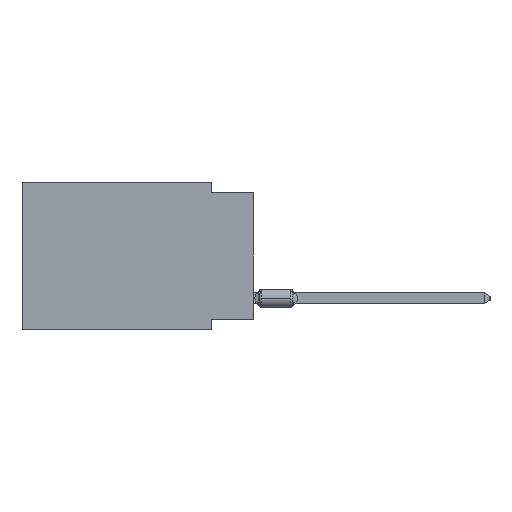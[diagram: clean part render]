
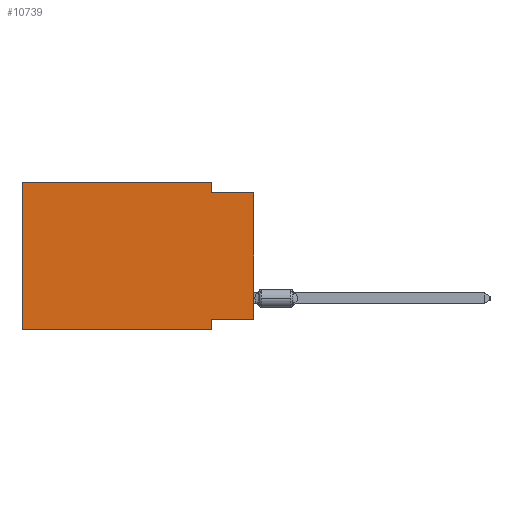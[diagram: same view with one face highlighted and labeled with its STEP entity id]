
A CAD part, left-side view. The second image highlights one B-rep face of the part: STEP entity #10739.
In plain terms, the highlighted planar face has unit normal (-1, 0, 0).
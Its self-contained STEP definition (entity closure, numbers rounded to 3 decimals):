
#89 = EDGE_CURVE ( 'NONE', #37740, #52494, #34075, .T. ) ;
#1620 = VERTEX_POINT ( 'NONE', #48824 ) ;
#2549 = DIRECTION ( 'NONE',  ( 0., 0., -1. ) ) ;
#2616 = DIRECTION ( 'NONE',  ( 0., 1., 0. ) ) ;
#3438 = VECTOR ( 'NONE', #48054, 1000. ) ;
#3888 = LINE ( 'NONE', #55420, #17510 ) ;
#4563 = ORIENTED_EDGE ( 'NONE', *, *, #40846, .T. ) ;
#4579 = DIRECTION ( 'NONE',  ( 0., 0., 1. ) ) ;
#4786 = EDGE_CURVE ( 'NONE', #1620, #22868, #50699, .T. ) ;
#5917 = ORIENTED_EDGE ( 'NONE', *, *, #14715, .F. ) ;
#9304 = EDGE_LOOP ( 'NONE', ( #4563, #17468, #33522, #39789, #30002, #59952, #5917, #35940 ) ) ;
#9480 = VECTOR ( 'NONE', #9847, 1000. ) ;
#9700 = LINE ( 'NONE', #28296, #36802 ) ;
#9847 = DIRECTION ( 'NONE',  ( 0., 0., -1. ) ) ;
#10182 = CARTESIAN_POINT ( 'NONE',  ( 0., 13.97, -8.89 ) ) ;
#10471 = CARTESIAN_POINT ( 'NONE',  ( 0., 2.54, 0. ) ) ;
#10739 = ADVANCED_FACE ( 'NONE', ( #45367 ), #35446, .F. ) ;
#10779 = CARTESIAN_POINT ( 'NONE',  ( 0., 13.97, 0. ) ) ;
#11839 = DIRECTION ( 'NONE',  ( 1., 0., 0. ) ) ;
#14715 = EDGE_CURVE ( 'NONE', #22868, #53963, #22720, .T. ) ;
#15828 = EDGE_CURVE ( 'NONE', #37740, #53963, #25347, .T. ) ;
#17404 = CARTESIAN_POINT ( 'NONE',  ( 0., 13.97, 0. ) ) ;
#17440 = AXIS2_PLACEMENT_3D ( 'NONE', #17404, #11839, #2549 ) ;
#17464 = DIRECTION ( 'NONE',  ( 0., 0., -1. ) ) ;
#17468 = ORIENTED_EDGE ( 'NONE', *, *, #26777, .F. ) ;
#17510 = VECTOR ( 'NONE', #56039, 1000. ) ;
#22555 = CARTESIAN_POINT ( 'NONE',  ( 0., 2.54, 0. ) ) ;
#22720 = LINE ( 'NONE', #26766, #59843 ) ;
#22868 = VERTEX_POINT ( 'NONE', #36745 ) ;
#25347 = LINE ( 'NONE', #10182, #3438 ) ;
#26766 = CARTESIAN_POINT ( 'NONE',  ( 0., 2.54, -8.89 ) ) ;
#26777 = EDGE_CURVE ( 'NONE', #56768, #56970, #3888, .T. ) ;
#27705 = VECTOR ( 'NONE', #4579, 1000. ) ;
#28296 = CARTESIAN_POINT ( 'NONE',  ( 0., 0., 0. ) ) ;
#28320 = CARTESIAN_POINT ( 'NONE',  ( 0., 2.54, -8.89 ) ) ;
#30002 = ORIENTED_EDGE ( 'NONE', *, *, #89, .F. ) ;
#30354 = CARTESIAN_POINT ( 'NONE',  ( 0., 0., -0.635 ) ) ;
#31615 = EDGE_CURVE ( 'NONE', #52494, #43075, #58930, .T. ) ;
#32310 = CARTESIAN_POINT ( 'NONE',  ( 0., 13.97, -8.89 ) ) ;
#32887 = VECTOR ( 'NONE', #2616, 1000. ) ;
#33522 = ORIENTED_EDGE ( 'NONE', *, *, #43219, .F. ) ;
#33750 = LINE ( 'NONE', #10471, #9480 ) ;
#34075 = LINE ( 'NONE', #10779, #27705 ) ;
#34492 = CARTESIAN_POINT ( 'NONE',  ( 0., 13.97, 0. ) ) ;
#35446 = PLANE ( 'NONE',  #17440 ) ;
#35940 = ORIENTED_EDGE ( 'NONE', *, *, #4786, .F. ) ;
#36745 = CARTESIAN_POINT ( 'NONE',  ( 0., 2.54, -8.255 ) ) ;
#36802 = VECTOR ( 'NONE', #51909, 1000. ) ;
#37740 = VERTEX_POINT ( 'NONE', #32310 ) ;
#39789 = ORIENTED_EDGE ( 'NONE', *, *, #31615, .F. ) ;
#40846 = EDGE_CURVE ( 'NONE', #1620, #56970, #9700, .T. ) ;
#43075 = VERTEX_POINT ( 'NONE', #22555 ) ;
#43219 = EDGE_CURVE ( 'NONE', #43075, #56768, #33750, .T. ) ;
#44045 = CARTESIAN_POINT ( 'NONE',  ( 0., 13.97, 0. ) ) ;
#44649 = DIRECTION ( 'NONE',  ( 0., -1., 0. ) ) ;
#45367 = FACE_OUTER_BOUND ( 'NONE', #9304, .T. ) ;
#48054 = DIRECTION ( 'NONE',  ( 0., -1., 0. ) ) ;
#48824 = CARTESIAN_POINT ( 'NONE',  ( 0., 0., -8.255 ) ) ;
#49805 = VECTOR ( 'NONE', #44649, 1000. ) ;
#50699 = LINE ( 'NONE', #54756, #32887 ) ;
#51909 = DIRECTION ( 'NONE',  ( 0., 0., 1. ) ) ;
#52411 = CARTESIAN_POINT ( 'NONE',  ( 0., 2.54, -0.635 ) ) ;
#52494 = VERTEX_POINT ( 'NONE', #34492 ) ;
#53963 = VERTEX_POINT ( 'NONE', #28320 ) ;
#54756 = CARTESIAN_POINT ( 'NONE',  ( 0., 0., -8.255 ) ) ;
#55420 = CARTESIAN_POINT ( 'NONE',  ( 0., 0., -0.635 ) ) ;
#56039 = DIRECTION ( 'NONE',  ( 0., -1., 0. ) ) ;
#56768 = VERTEX_POINT ( 'NONE', #52411 ) ;
#56970 = VERTEX_POINT ( 'NONE', #30354 ) ;
#58930 = LINE ( 'NONE', #44045, #49805 ) ;
#59843 = VECTOR ( 'NONE', #17464, 1000. ) ;
#59952 = ORIENTED_EDGE ( 'NONE', *, *, #15828, .T. ) ;
